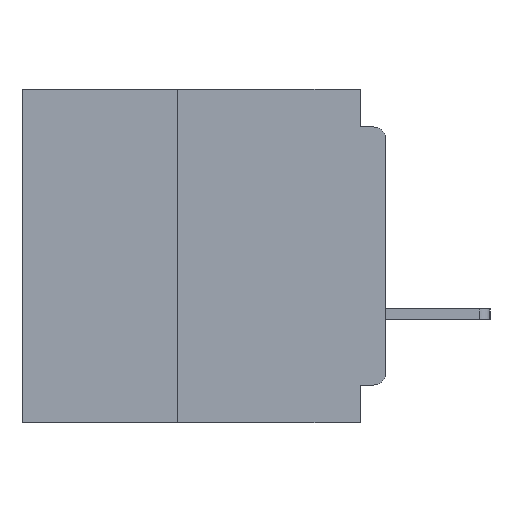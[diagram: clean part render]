
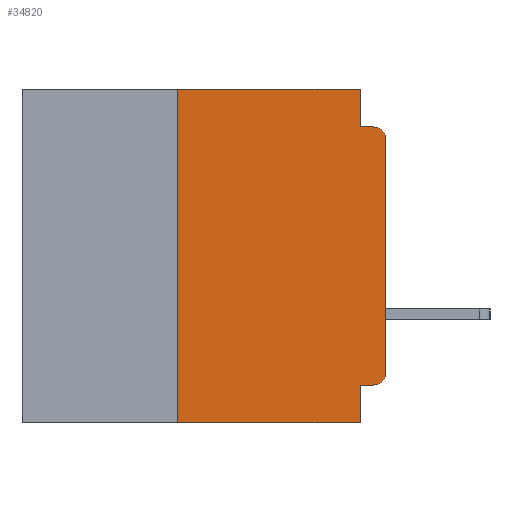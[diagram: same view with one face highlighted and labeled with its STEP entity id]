
A CAD part, left-side view. The second image highlights one B-rep face of the part: STEP entity #34820.
In plain terms, the highlighted planar face has unit normal (-1, 0, 0).
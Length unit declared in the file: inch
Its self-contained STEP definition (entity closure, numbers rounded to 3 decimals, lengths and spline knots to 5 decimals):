
#2134 = LINE ( 'NONE', #37851, #12467 ) ;
#4228 = ORIENTED_EDGE ( 'NONE', *, *, #58904, .F. ) ;
#4883 = AXIS2_PLACEMENT_3D ( 'NONE', #39781, #9770, #44828 ) ;
#5875 = ORIENTED_EDGE ( 'NONE', *, *, #47661, .F. ) ;
#5876 = ORIENTED_EDGE ( 'NONE', *, *, #39244, .T. ) ;
#6227 = EDGE_CURVE ( 'NONE', #12524, #46240, #17592, .T. ) ;
#7213 = CARTESIAN_POINT ( 'NONE',  ( 0., 0.031, -0.4 ) ) ;
#8471 = CARTESIAN_POINT ( 'NONE',  ( 0., 0.015, -0.045 ) ) ;
#9770 = DIRECTION ( 'NONE',  ( 1., 0., 0. ) ) ;
#11179 = ORIENTED_EDGE ( 'NONE', *, *, #12716, .T. ) ;
#11599 = VERTEX_POINT ( 'NONE', #15000 ) ;
#11658 = DIRECTION ( 'NONE',  ( 0., 0., 1. ) ) ;
#12005 = EDGE_CURVE ( 'NONE', #31814, #20555, #64010, .T. ) ;
#12467 = VECTOR ( 'NONE', #47685, 39.37008 ) ;
#12524 = VERTEX_POINT ( 'NONE', #22541 ) ;
#12716 = EDGE_CURVE ( 'NONE', #32152, #12524, #46512, .T. ) ;
#12811 = LINE ( 'NONE', #17794, #63064 ) ;
#13030 = CARTESIAN_POINT ( 'NONE',  ( 0., 0.015, -0.06 ) ) ;
#14524 = CIRCLE ( 'NONE', #50054, 0.015 ) ;
#15000 = CARTESIAN_POINT ( 'NONE',  ( 0., 0.031, 0. ) ) ;
#15229 = EDGE_CURVE ( 'NONE', #63539, #31814, #2134, .T. ) ;
#16069 = EDGE_CURVE ( 'NONE', #38530, #20555, #25678, .T. ) ;
#16584 = VERTEX_POINT ( 'NONE', #35863 ) ;
#17592 = CIRCLE ( 'NONE', #65145, 0.015 ) ;
#17794 = CARTESIAN_POINT ( 'NONE',  ( 0., 0.031, 0. ) ) ;
#18072 = DIRECTION ( 'NONE',  ( 0., 0., -1. ) ) ;
#18478 = DIRECTION ( 'NONE',  ( 0., 0., -1. ) ) ;
#19446 = FACE_OUTER_BOUND ( 'NONE', #34567, .T. ) ;
#19911 = VECTOR ( 'NONE', #11658, 39.37008 ) ;
#20555 = VERTEX_POINT ( 'NONE', #7213 ) ;
#20924 = DIRECTION ( 'NONE',  ( -1., 0., 0. ) ) ;
#22457 = EDGE_CURVE ( 'NONE', #16584, #11599, #41978, .T. ) ;
#22541 = CARTESIAN_POINT ( 'NONE',  ( 0., 0., -0.06 ) ) ;
#22629 = CARTESIAN_POINT ( 'NONE',  ( 0., 0.25, -0.4 ) ) ;
#22790 = DIRECTION ( 'NONE',  ( 0., 0., -1. ) ) ;
#23291 = CARTESIAN_POINT ( 'NONE',  ( 0., 0.437, 0. ) ) ;
#23558 = CARTESIAN_POINT ( 'NONE',  ( 0., 0.015, -0.355 ) ) ;
#24745 = CARTESIAN_POINT ( 'NONE',  ( 0., 0.25, -0.4 ) ) ;
#25678 = LINE ( 'NONE', #26922, #52348 ) ;
#26922 = CARTESIAN_POINT ( 'NONE',  ( 0., 0.437, -0.4 ) ) ;
#29673 = VECTOR ( 'NONE', #47793, 39.37008 ) ;
#29775 = PLANE ( 'NONE',  #4883 ) ;
#31814 = VERTEX_POINT ( 'NONE', #32346 ) ;
#32144 = VECTOR ( 'NONE', #58909, 39.37008 ) ;
#32152 = VERTEX_POINT ( 'NONE', #65237 ) ;
#32346 = CARTESIAN_POINT ( 'NONE',  ( 0., 0.031, -0.355 ) ) ;
#34567 = EDGE_LOOP ( 'NONE', ( #11179, #56325, #4228, #47858, #44592, #5875, #40013, #58730, #40078, #5876 ) ) ;
#34820 = ADVANCED_FACE ( 'NONE', ( #19446 ), #29775, .F. ) ;
#35863 = CARTESIAN_POINT ( 'NONE',  ( 0., 0.25, 0. ) ) ;
#36644 = CARTESIAN_POINT ( 'NONE',  ( 0., 0., 0. ) ) ;
#37851 = CARTESIAN_POINT ( 'NONE',  ( 0., 0., -0.355 ) ) ;
#38530 = VERTEX_POINT ( 'NONE', #24745 ) ;
#39244 = EDGE_CURVE ( 'NONE', #63539, #32152, #14524, .T. ) ;
#39265 = VERTEX_POINT ( 'NONE', #45854 ) ;
#39781 = CARTESIAN_POINT ( 'NONE',  ( 0., 0.437, 0. ) ) ;
#40013 = ORIENTED_EDGE ( 'NONE', *, *, #16069, .T. ) ;
#40078 = ORIENTED_EDGE ( 'NONE', *, *, #15229, .F. ) ;
#40420 = VECTOR ( 'NONE', #63473, 39.37008 ) ;
#41978 = LINE ( 'NONE', #23291, #40420 ) ;
#42916 = LINE ( 'NONE', #22629, #29673 ) ;
#44592 = ORIENTED_EDGE ( 'NONE', *, *, #22457, .F. ) ;
#44828 = DIRECTION ( 'NONE',  ( 0., 0., -1. ) ) ;
#45854 = CARTESIAN_POINT ( 'NONE',  ( 0., 0.031, -0.045 ) ) ;
#46240 = VERTEX_POINT ( 'NONE', #8471 ) ;
#46512 = LINE ( 'NONE', #36644, #19911 ) ;
#47661 = EDGE_CURVE ( 'NONE', #38530, #16584, #42916, .T. ) ;
#47685 = DIRECTION ( 'NONE',  ( 0., 1., 0. ) ) ;
#47793 = DIRECTION ( 'NONE',  ( 0., 0., 1. ) ) ;
#47858 = ORIENTED_EDGE ( 'NONE', *, *, #56937, .F. ) ;
#48035 = DIRECTION ( 'NONE',  ( -1., 0., 0. ) ) ;
#48446 = CARTESIAN_POINT ( 'NONE',  ( 0., 0.031, -0.4 ) ) ;
#50054 = AXIS2_PLACEMENT_3D ( 'NONE', #50922, #20924, #56036 ) ;
#50922 = CARTESIAN_POINT ( 'NONE',  ( 0., 0.015, -0.34 ) ) ;
#52167 = VECTOR ( 'NONE', #18478, 39.37008 ) ;
#52348 = VECTOR ( 'NONE', #62090, 39.37008 ) ;
#56036 = DIRECTION ( 'NONE',  ( 0., 0., -1. ) ) ;
#56325 = ORIENTED_EDGE ( 'NONE', *, *, #6227, .T. ) ;
#56937 = EDGE_CURVE ( 'NONE', #11599, #39265, #12811, .T. ) ;
#58696 = CARTESIAN_POINT ( 'NONE',  ( 0., 0., -0.045 ) ) ;
#58730 = ORIENTED_EDGE ( 'NONE', *, *, #12005, .F. ) ;
#58904 = EDGE_CURVE ( 'NONE', #39265, #46240, #60445, .T. ) ;
#58909 = DIRECTION ( 'NONE',  ( 0., -1., 0. ) ) ;
#60445 = LINE ( 'NONE', #58696, #32144 ) ;
#62090 = DIRECTION ( 'NONE',  ( 0., -1., 0. ) ) ;
#63064 = VECTOR ( 'NONE', #22790, 39.37008 ) ;
#63473 = DIRECTION ( 'NONE',  ( 0., -1., 0. ) ) ;
#63539 = VERTEX_POINT ( 'NONE', #23558 ) ;
#64010 = LINE ( 'NONE', #48446, #52167 ) ;
#65145 = AXIS2_PLACEMENT_3D ( 'NONE', #13030, #48035, #18072 ) ;
#65237 = CARTESIAN_POINT ( 'NONE',  ( 0., 0., -0.34 ) ) ;
